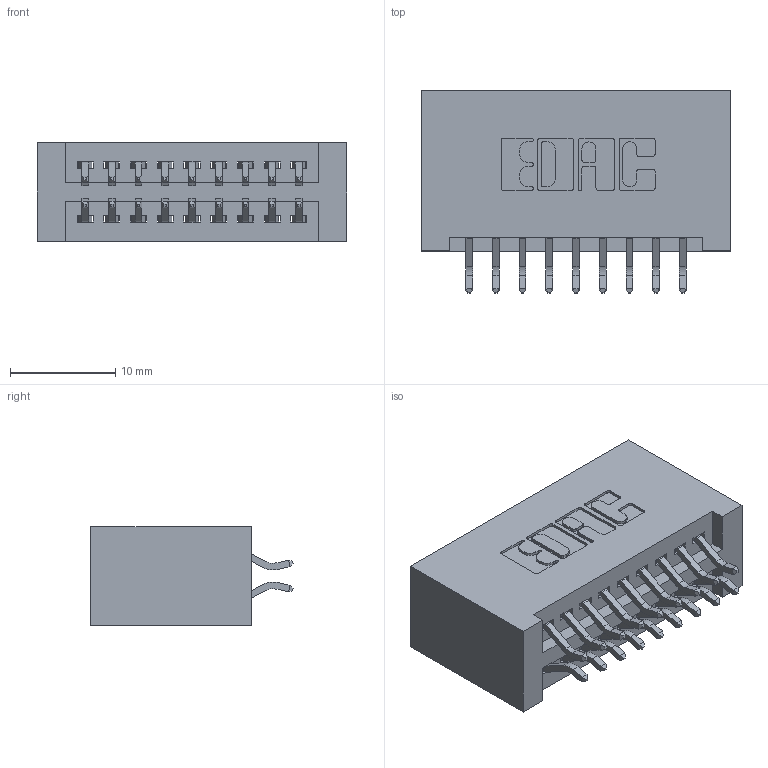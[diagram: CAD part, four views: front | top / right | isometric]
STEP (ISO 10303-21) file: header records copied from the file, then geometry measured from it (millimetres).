
FILE_DESCRIPTION (( 'STEP AP203' ), '1' );
FILE_NAME ('345-018-556-201.STEP', '2019-10-27T06:49:03', ( '' ), ( '' ), 'SwSTEP 2.0', 'SolidWorks 2016', '' );
FILE_SCHEMA (( 'CONFIG_CONTROL_DESIGN' ));
Length unit declared in the file: inch
Products named in the file (3): 345-292-001_556 Tail; 345-018-556-201; 345 Part_No Mounting Lugs
Assembly tree (19 placements, depth 2):
  345-018-556-201
    345 Part_No Mounting Lugs
    345-292-001_556 Tail  x18
Bounding box: 29.46 x 19.24 x 9.4 mm (x, y, z)
Volume: 3171 mm3; surface area: 4335.7 mm2
Topology: 19 solids, 19 shells, 1126 faces, 3323 edges, 2190 vertices
Faces by surface type: plane 742, cylinder 384
Entity records: 11447 total; most frequent: CARTESIAN_POINT 1964, ORIENTED_EDGE 1886, DIRECTION 1755, EDGE_CURVE 943, VECTOR 775, LINE 775, VERTEX_POINT 626, AXIS2_PLACEMENT_3D 490
